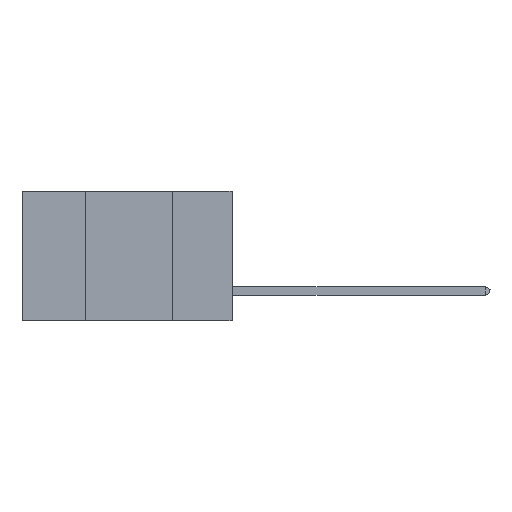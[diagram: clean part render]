
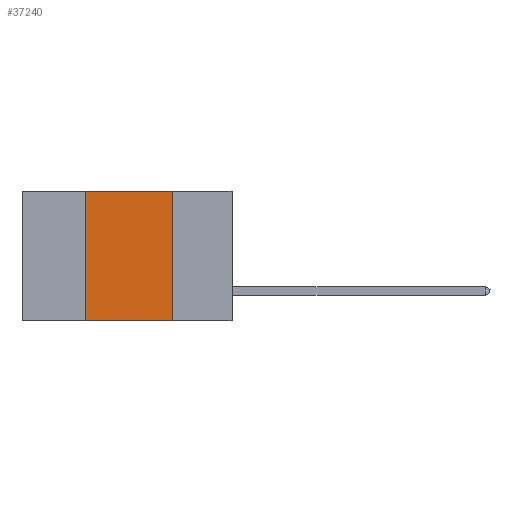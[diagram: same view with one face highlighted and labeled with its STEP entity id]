
A CAD part, left-side view. The second image highlights one B-rep face of the part: STEP entity #37240.
In plain terms, the highlighted planar face has unit normal (-1, 0, 0).
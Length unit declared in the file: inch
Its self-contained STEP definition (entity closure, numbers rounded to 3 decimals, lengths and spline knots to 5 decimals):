
#2916 = DIRECTION ( 'NONE',  ( 0., 0., -1. ) ) ;
#4219 = VERTEX_POINT ( 'NONE', #22504 ) ;
#4351 = CARTESIAN_POINT ( 'NONE',  ( 0., 0.17, 0. ) ) ;
#5087 = VERTEX_POINT ( 'NONE', #27531 ) ;
#6064 = CARTESIAN_POINT ( 'NONE',  ( 0., 0.42, -0.37 ) ) ;
#8776 = EDGE_LOOP ( 'NONE', ( #29859, #27911, #30422, #13938 ) ) ;
#9433 = AXIS2_PLACEMENT_3D ( 'NONE', #41935, #22425, #2916 ) ;
#13290 = VECTOR ( 'NONE', #30730, 39.37008 ) ;
#13938 = ORIENTED_EDGE ( 'NONE', *, *, #22557, .T. ) ;
#14401 = VECTOR ( 'NONE', #39584, 39.37008 ) ;
#15396 = CARTESIAN_POINT ( 'NONE',  ( 0., 0.6, -0.37 ) ) ;
#15910 = LINE ( 'NONE', #4351, #13290 ) ;
#19711 = EDGE_CURVE ( 'NONE', #4219, #27830, #39304, .T. ) ;
#20501 = LINE ( 'NONE', #37351, #28689 ) ;
#22425 = DIRECTION ( 'NONE',  ( 1., 0., 0. ) ) ;
#22504 = CARTESIAN_POINT ( 'NONE',  ( 0., 0.42, 0. ) ) ;
#22557 = EDGE_CURVE ( 'NONE', #25371, #5087, #27899, .T. ) ;
#23690 = CARTESIAN_POINT ( 'NONE',  ( 0., 0.6, 0. ) ) ;
#25371 = VERTEX_POINT ( 'NONE', #6064 ) ;
#26995 = DIRECTION ( 'NONE',  ( 0., 0., 1. ) ) ;
#27531 = CARTESIAN_POINT ( 'NONE',  ( 0., 0.17, -0.37 ) ) ;
#27830 = VERTEX_POINT ( 'NONE', #31438 ) ;
#27899 = LINE ( 'NONE', #15396, #42143 ) ;
#27911 = ORIENTED_EDGE ( 'NONE', *, *, #19711, .F. ) ;
#28689 = VECTOR ( 'NONE', #26995, 39.37008 ) ;
#29859 = ORIENTED_EDGE ( 'NONE', *, *, #34478, .F. ) ;
#30422 = ORIENTED_EDGE ( 'NONE', *, *, #34014, .F. ) ;
#30730 = DIRECTION ( 'NONE',  ( 0., 0., -1. ) ) ;
#31438 = CARTESIAN_POINT ( 'NONE',  ( 0., 0.17, 0. ) ) ;
#34014 = EDGE_CURVE ( 'NONE', #25371, #4219, #20501, .T. ) ;
#34478 = EDGE_CURVE ( 'NONE', #27830, #5087, #15910, .T. ) ;
#37240 = ADVANCED_FACE ( 'NONE', ( #40795 ), #38625, .F. ) ;
#37351 = CARTESIAN_POINT ( 'NONE',  ( 0., 0.42, 0. ) ) ;
#38153 = DIRECTION ( 'NONE',  ( 0., -1., 0. ) ) ;
#38625 = PLANE ( 'NONE',  #9433 ) ;
#39304 = LINE ( 'NONE', #23690, #14401 ) ;
#39584 = DIRECTION ( 'NONE',  ( 0., -1., 0. ) ) ;
#40795 = FACE_OUTER_BOUND ( 'NONE', #8776, .T. ) ;
#41935 = CARTESIAN_POINT ( 'NONE',  ( 0., 0.6, 0. ) ) ;
#42143 = VECTOR ( 'NONE', #38153, 39.37008 ) ;
